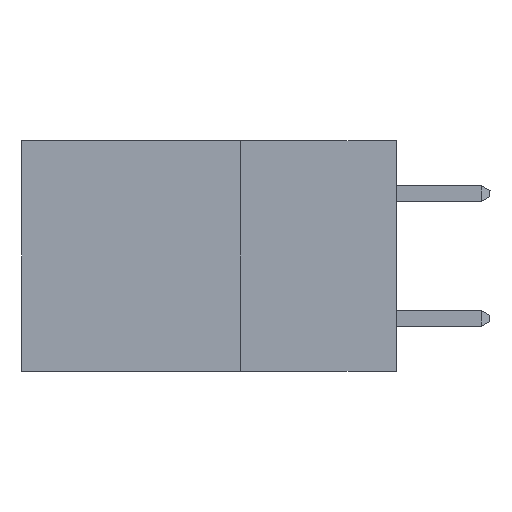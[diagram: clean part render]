
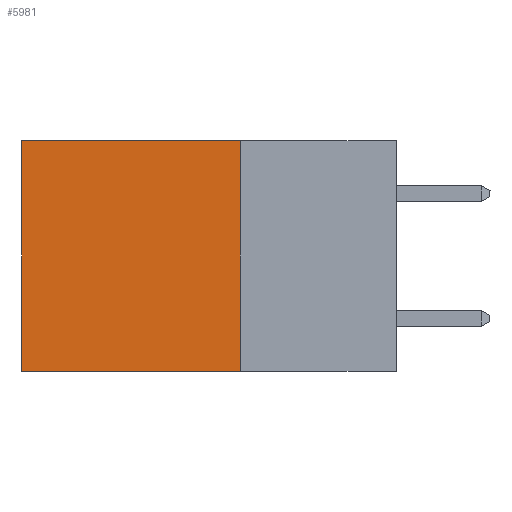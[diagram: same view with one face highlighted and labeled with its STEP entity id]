
A CAD part, left-side view. The second image highlights one B-rep face of the part: STEP entity #5981.
In plain terms, the highlighted planar face has unit normal (-1, 0, 0).
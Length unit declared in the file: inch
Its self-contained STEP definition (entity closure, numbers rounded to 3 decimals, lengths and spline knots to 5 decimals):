
#317 = DIRECTION ( 'NONE',  ( 0., 0., -1. ) ) ;
#950 = LINE ( 'NONE', #3275, #2033 ) ;
#1324 = CARTESIAN_POINT ( 'NONE',  ( 0.298, 0.6, -0.37 ) ) ;
#1377 = ORIENTED_EDGE ( 'NONE', *, *, #5422, .T. ) ;
#1599 = ORIENTED_EDGE ( 'NONE', *, *, #5999, .F. ) ;
#1994 = VERTEX_POINT ( 'NONE', #4350 ) ;
#2033 = VECTOR ( 'NONE', #317, 39.37008 ) ;
#2340 = LINE ( 'NONE', #4891, #9201 ) ;
#2673 = PLANE ( 'NONE',  #8660 ) ;
#2996 = CARTESIAN_POINT ( 'NONE',  ( 0.298, 0.6, 0. ) ) ;
#3029 = EDGE_CURVE ( 'NONE', #1994, #6158, #2340, .T. ) ;
#3241 = LINE ( 'NONE', #4728, #6982 ) ;
#3264 = CARTESIAN_POINT ( 'NONE',  ( 0.298, 0.25, 0. ) ) ;
#3275 = CARTESIAN_POINT ( 'NONE',  ( 0.298, 0.25, 0. ) ) ;
#3742 = ORIENTED_EDGE ( 'NONE', *, *, #3029, .F. ) ;
#4257 = DIRECTION ( 'NONE',  ( 0., 0., -1. ) ) ;
#4350 = CARTESIAN_POINT ( 'NONE',  ( 0.298, 0.25, -0.37 ) ) ;
#4700 = EDGE_LOOP ( 'NONE', ( #1377, #3742, #1599, #7328 ) ) ;
#4707 = DIRECTION ( 'NONE',  ( 0., 1., 0. ) ) ;
#4728 = CARTESIAN_POINT ( 'NONE',  ( 0.298, 0.25, 0. ) ) ;
#4891 = CARTESIAN_POINT ( 'NONE',  ( 0.298, 0.25, -0.37 ) ) ;
#5208 = VECTOR ( 'NONE', #4257, 39.37008 ) ;
#5422 = EDGE_CURVE ( 'NONE', #9158, #6158, #7009, .T. ) ;
#5500 = VERTEX_POINT ( 'NONE', #8385 ) ;
#5515 = DIRECTION ( 'NONE',  ( 0., 0., -1. ) ) ;
#5803 = DIRECTION ( 'NONE',  ( 1., 0., 0. ) ) ;
#5981 = ADVANCED_FACE ( 'NONE', ( #6153 ), #2673, .F. ) ;
#5999 = EDGE_CURVE ( 'NONE', #5500, #1994, #950, .T. ) ;
#6153 = FACE_OUTER_BOUND ( 'NONE', #4700, .T. ) ;
#6158 = VERTEX_POINT ( 'NONE', #1324 ) ;
#6594 = EDGE_CURVE ( 'NONE', #5500, #9158, #3241, .T. ) ;
#6982 = VECTOR ( 'NONE', #4707, 39.37008 ) ;
#7009 = LINE ( 'NONE', #9069, #5208 ) ;
#7328 = ORIENTED_EDGE ( 'NONE', *, *, #6594, .T. ) ;
#8254 = DIRECTION ( 'NONE',  ( 0., 1., 0. ) ) ;
#8385 = CARTESIAN_POINT ( 'NONE',  ( 0.298, 0.25, 0. ) ) ;
#8660 = AXIS2_PLACEMENT_3D ( 'NONE', #3264, #5803, #5515 ) ;
#9069 = CARTESIAN_POINT ( 'NONE',  ( 0.298, 0.6, 0. ) ) ;
#9158 = VERTEX_POINT ( 'NONE', #2996 ) ;
#9201 = VECTOR ( 'NONE', #8254, 39.37008 ) ;
